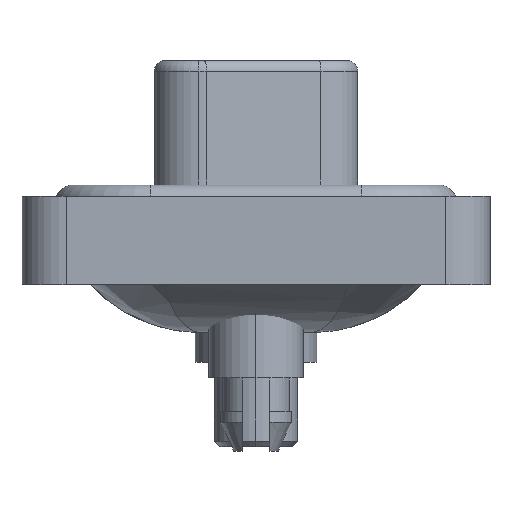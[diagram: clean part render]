
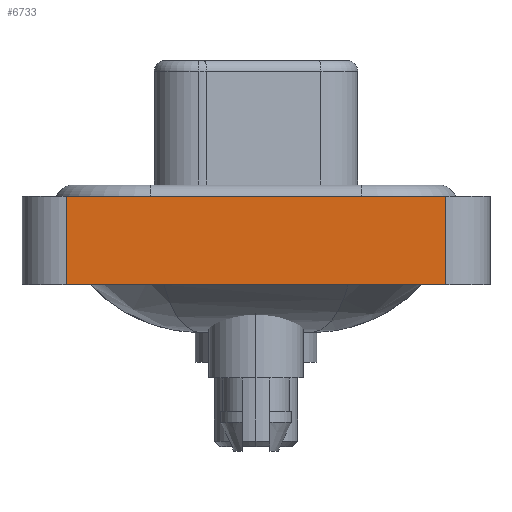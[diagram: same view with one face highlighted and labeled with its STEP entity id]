
A CAD part, left-side view. The second image highlights one B-rep face of the part: STEP entity #6733.
In plain terms, the highlighted planar face has unit normal (-1, 0, 0).
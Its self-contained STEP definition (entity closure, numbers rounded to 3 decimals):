
#944 = CARTESIAN_POINT ( 'NONE',  ( -7.25, -8.55, -3.6 ) ) ;
#1498 = DIRECTION ( 'NONE',  ( 0., 0., 1. ) ) ;
#1761 = LINE ( 'NONE', #22619, #22375 ) ;
#3033 = DIRECTION ( 'NONE',  ( 0., 0., 1. ) ) ;
#3285 = EDGE_CURVE ( 'NONE', #7421, #9901, #1761, .T. ) ;
#3367 = EDGE_CURVE ( 'NONE', #8488, #7421, #5227, .T. ) ;
#3762 = CARTESIAN_POINT ( 'NONE',  ( -7.25, -8.55, -3.6 ) ) ;
#4089 = CARTESIAN_POINT ( 'NONE',  ( -7.25, -8.55, -3.6 ) ) ;
#5227 = LINE ( 'NONE', #17338, #6581 ) ;
#6581 = VECTOR ( 'NONE', #1498, 1000. ) ;
#6733 = ADVANCED_FACE ( 'NONE', ( #10947 ), #18072, .T. ) ;
#6878 = DIRECTION ( 'NONE',  ( 0., -1., 0. ) ) ;
#7250 = DIRECTION ( 'NONE',  ( -1., 0., 0. ) ) ;
#7421 = VERTEX_POINT ( 'NONE', #18962 ) ;
#8488 = VERTEX_POINT ( 'NONE', #11240 ) ;
#8871 = CARTESIAN_POINT ( 'NONE',  ( -7.25, -8.55, -3.6 ) ) ;
#8989 = DIRECTION ( 'NONE',  ( 0., 0., 1. ) ) ;
#9301 = ORIENTED_EDGE ( 'NONE', *, *, #17817, .T. ) ;
#9901 = VERTEX_POINT ( 'NONE', #18880 ) ;
#10825 = VERTEX_POINT ( 'NONE', #4089 ) ;
#10947 = FACE_OUTER_BOUND ( 'NONE', #20203, .T. ) ;
#11240 = CARTESIAN_POINT ( 'NONE',  ( -7.25, 8.55, -3.6 ) ) ;
#13035 = AXIS2_PLACEMENT_3D ( 'NONE', #3762, #7250, #8989 ) ;
#15132 = ORIENTED_EDGE ( 'NONE', *, *, #3367, .F. ) ;
#15435 = ORIENTED_EDGE ( 'NONE', *, *, #22410, .T. ) ;
#15593 = VECTOR ( 'NONE', #15885, 1000. ) ;
#15885 = DIRECTION ( 'NONE',  ( 0., -1., 0. ) ) ;
#17125 = LINE ( 'NONE', #944, #22120 ) ;
#17338 = CARTESIAN_POINT ( 'NONE',  ( -7.25, 8.55, -3.6 ) ) ;
#17619 = LINE ( 'NONE', #8871, #15593 ) ;
#17817 = EDGE_CURVE ( 'NONE', #10825, #9901, #17125, .T. ) ;
#18072 = PLANE ( 'NONE',  #13035 ) ;
#18880 = CARTESIAN_POINT ( 'NONE',  ( -7.25, -8.55, 0.4 ) ) ;
#18962 = CARTESIAN_POINT ( 'NONE',  ( -7.25, 8.55, 0.4 ) ) ;
#19160 = ORIENTED_EDGE ( 'NONE', *, *, #3285, .F. ) ;
#20203 = EDGE_LOOP ( 'NONE', ( #9301, #19160, #15132, #15435 ) ) ;
#22120 = VECTOR ( 'NONE', #3033, 1000. ) ;
#22375 = VECTOR ( 'NONE', #6878, 1000. ) ;
#22410 = EDGE_CURVE ( 'NONE', #8488, #10825, #17619, .T. ) ;
#22619 = CARTESIAN_POINT ( 'NONE',  ( -7.25, -8.55, 0.4 ) ) ;
